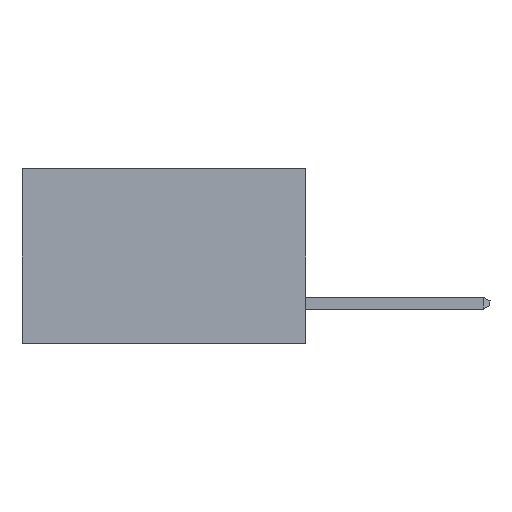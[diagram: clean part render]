
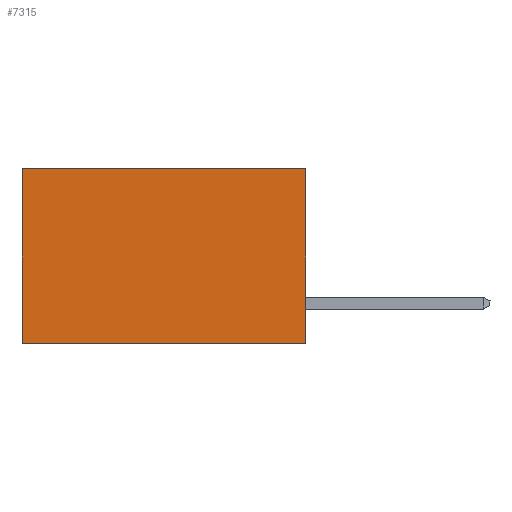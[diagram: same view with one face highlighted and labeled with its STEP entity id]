
A CAD part, left-side view. The second image highlights one B-rep face of the part: STEP entity #7315.
In plain terms, the highlighted planar face has unit normal (-1, 0, 0).
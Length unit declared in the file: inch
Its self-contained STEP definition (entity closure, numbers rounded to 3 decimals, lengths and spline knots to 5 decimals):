
#7 = VECTOR ( 'NONE', #3596, 39.37008 ) ;
#395 = VECTOR ( 'NONE', #5890, 39.37008 ) ;
#994 = VERTEX_POINT ( 'NONE', #6180 ) ;
#1212 = DIRECTION ( 'NONE',  ( 1., 0., 0. ) ) ;
#1226 = EDGE_CURVE ( 'NONE', #3022, #1860, #4617, .T. ) ;
#1366 = ORIENTED_EDGE ( 'NONE', *, *, #1226, .F. ) ;
#1571 = EDGE_LOOP ( 'NONE', ( #1777, #3684, #1366, #3074 ) ) ;
#1773 = VECTOR ( 'NONE', #5524, 39.37008 ) ;
#1777 = ORIENTED_EDGE ( 'NONE', *, *, #2855, .T. ) ;
#1842 = CARTESIAN_POINT ( 'NONE',  ( 0.2615, 0., 0. ) ) ;
#1860 = VERTEX_POINT ( 'NONE', #4054 ) ;
#2496 = EDGE_CURVE ( 'NONE', #1860, #994, #5478, .T. ) ;
#2625 = FACE_OUTER_BOUND ( 'NONE', #1571, .T. ) ;
#2684 = AXIS2_PLACEMENT_3D ( 'NONE', #5327, #1212, #6671 ) ;
#2855 = EDGE_CURVE ( 'NONE', #4910, #994, #4151, .T. ) ;
#3022 = VERTEX_POINT ( 'NONE', #5156 ) ;
#3074 = ORIENTED_EDGE ( 'NONE', *, *, #7321, .T. ) ;
#3596 = DIRECTION ( 'NONE',  ( 0., 0., -1. ) ) ;
#3684 = ORIENTED_EDGE ( 'NONE', *, *, #2496, .F. ) ;
#4054 = CARTESIAN_POINT ( 'NONE',  ( 0.2615, 0., -0.37 ) ) ;
#4151 = LINE ( 'NONE', #7498, #7 ) ;
#4617 = LINE ( 'NONE', #5318, #395 ) ;
#4910 = VERTEX_POINT ( 'NONE', #5734 ) ;
#5156 = CARTESIAN_POINT ( 'NONE',  ( 0.2615, 0., 0. ) ) ;
#5318 = CARTESIAN_POINT ( 'NONE',  ( 0.2615, 0., -0.37 ) ) ;
#5327 = CARTESIAN_POINT ( 'NONE',  ( 0.2615, 0., -0.37 ) ) ;
#5478 = LINE ( 'NONE', #7522, #1773 ) ;
#5524 = DIRECTION ( 'NONE',  ( 0., 1., 0. ) ) ;
#5734 = CARTESIAN_POINT ( 'NONE',  ( 0.2615, 0.6, 0. ) ) ;
#5890 = DIRECTION ( 'NONE',  ( 0., 0., -1. ) ) ;
#6180 = CARTESIAN_POINT ( 'NONE',  ( 0.2615, 0.6, -0.37 ) ) ;
#6508 = PLANE ( 'NONE',  #2684 ) ;
#6671 = DIRECTION ( 'NONE',  ( 0., 0., -1. ) ) ;
#7272 = DIRECTION ( 'NONE',  ( 0., 1., 0. ) ) ;
#7315 = ADVANCED_FACE ( 'NONE', ( #2625 ), #6508, .F. ) ;
#7321 = EDGE_CURVE ( 'NONE', #3022, #4910, #8498, .T. ) ;
#7498 = CARTESIAN_POINT ( 'NONE',  ( 0.2615, 0.6, -0.37 ) ) ;
#7522 = CARTESIAN_POINT ( 'NONE',  ( 0.2615, 0., -0.37 ) ) ;
#7552 = VECTOR ( 'NONE', #7272, 39.37008 ) ;
#8498 = LINE ( 'NONE', #1842, #7552 ) ;
